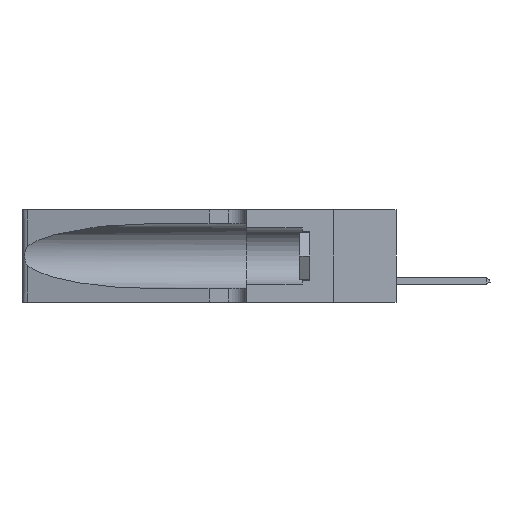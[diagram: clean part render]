
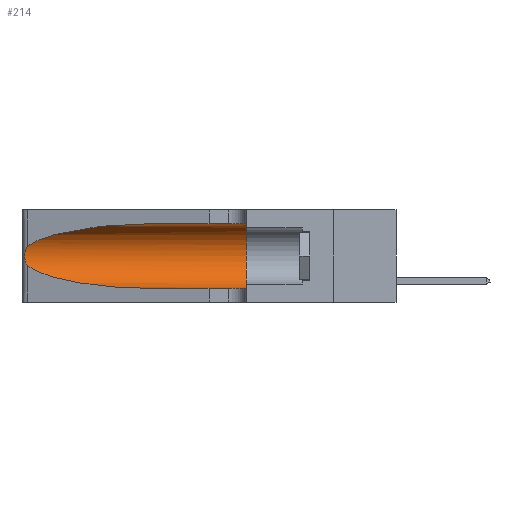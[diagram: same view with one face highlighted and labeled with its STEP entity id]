
A CAD part, left-side view. The second image highlights one B-rep face of the part: STEP entity #214.
In plain terms, the highlighted cylindrical face has radius 3.308 mm (diameter 6.617 mm), a partial arc.
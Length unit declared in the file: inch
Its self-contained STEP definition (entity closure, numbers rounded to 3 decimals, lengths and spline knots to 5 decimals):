
#214 = ADVANCED_FACE ( 'NONE', ( #5492 ), #4150, .F. ) ;
#510 = DIRECTION ( 'NONE',  ( 0., -1., 0. ) ) ;
#840 = CARTESIAN_POINT ( 'NONE',  ( 0.1305, 1.61858, 0.185 ) ) ;
#856 = VECTOR ( 'NONE', #5465, 39.37008 ) ;
#900 = ORIENTED_EDGE ( 'NONE', *, *, #8862, .F. ) ;
#1445 = ORIENTED_EDGE ( 'NONE', *, *, #20544, .T. ) ;
#1498 = AXIS2_PLACEMENT_3D ( 'NONE', #840, #18114, #11240 ) ;
#1716 = ORIENTED_EDGE ( 'NONE', *, *, #21447, .T. ) ;
#1896 = CARTESIAN_POINT ( 'NONE',  ( 0.1305, 1.61858, 0.05475 ) ) ;
#2707 = CARTESIAN_POINT ( 'NONE',  ( 0.25487, 1.22718, 0.14631 ) ) ;
#2871 = ORIENTED_EDGE ( 'NONE', *, *, #12090, .T. ) ;
#3190 = CARTESIAN_POINT ( 'NONE',  ( 0.25639, 1.23184, 0.21858 ) ) ;
#3364 =( BOUNDED_CURVE ( )  B_SPLINE_CURVE ( 3, ( #4228, #4074, #5873, #16490 ),
 .UNSPECIFIED., .F., .F. ) 
 B_SPLINE_CURVE_WITH_KNOTS ( ( 4, 4 ),
 ( 1.5708, 2.84003 ),
 .UNSPECIFIED. ) 
 CURVE ( )  GEOMETRIC_REPRESENTATION_ITEM ( )  RATIONAL_B_SPLINE_CURVE ( ( 1., 0.87, 0.87, 1. ) ) 
 REPRESENTATION_ITEM ( '' )  );
#3707 = CARTESIAN_POINT ( 'NONE',  ( 0.1305, 1.61858, 0.31525 ) ) ;
#4074 = CARTESIAN_POINT ( 'NONE',  ( 0.18966, 0.96281, 0.31525 ) ) ;
#4150 = CYLINDRICAL_SURFACE ( 'NONE', #1498, 0.13025 ) ;
#4228 = CARTESIAN_POINT ( 'NONE',  ( 0.1305, 0.72297, 0.31525 ) ) ;
#5065 = EDGE_CURVE ( 'NONE', #10031, #9863, #18889, .T. ) ;
#5465 = DIRECTION ( 'NONE',  ( 0., -1., 0. ) ) ;
#5492 = FACE_OUTER_BOUND ( 'NONE', #17828, .T. ) ;
#5762 = CARTESIAN_POINT ( 'NONE',  ( 0.1305, 0.35, 0.05475 ) ) ;
#5873 = CARTESIAN_POINT ( 'NONE',  ( 0.2373, 1.15595, 0.28018 ) ) ;
#6160 = CARTESIAN_POINT ( 'NONE',  ( 0.18966, 0.96281, 0.05475 ) ) ;
#6528 = LINE ( 'NONE', #1896, #17446 ) ;
#6623 = CARTESIAN_POINT ( 'NONE',  ( 0.26075, 1.23896, 0.178 ) ) ;
#8283 = CARTESIAN_POINT ( 'NONE',  ( 0.26018, 1.23835, 0.19895 ) ) ;
#8862 = EDGE_CURVE ( 'NONE', #9041, #10031, #13984, .T. ) ;
#9041 = VERTEX_POINT ( 'NONE', #22423 ) ;
#9112 = VERTEX_POINT ( 'NONE', #22352 ) ;
#9363 = VERTEX_POINT ( 'NONE', #14902 ) ;
#9863 = VERTEX_POINT ( 'NONE', #5762 ) ;
#10031 = VERTEX_POINT ( 'NONE', #20386 ) ;
#10655 = CARTESIAN_POINT ( 'NONE',  ( 0.25487, 1.22718, 0.22369 ) ) ;
#11240 = DIRECTION ( 'NONE',  ( 0., 0., -1. ) ) ;
#11399 = CARTESIAN_POINT ( 'NONE',  ( 0.2373, 1.15595, 0.08982 ) ) ;
#11960 = CARTESIAN_POINT ( 'NONE',  ( 0.25854, 1.2359, 0.20912 ) ) ;
#12090 = EDGE_CURVE ( 'NONE', #9041, #21643, #3364, .T. ) ;
#12695 = EDGE_CURVE ( 'NONE', #9363, #9112, #14134, .T. ) ;
#13054 = ORIENTED_EDGE ( 'NONE', *, *, #12695, .T. ) ;
#13269 = AXIS2_PLACEMENT_3D ( 'NONE', #20244, #19953, #22346 ) ;
#13403 = CARTESIAN_POINT ( 'NONE',  ( 0.25639, 1.23186, 0.15144 ) ) ;
#13471 = CARTESIAN_POINT ( 'NONE',  ( 0.25487, 1.22718, 0.14631 ) ) ;
#13553 = ORIENTED_EDGE ( 'NONE', *, *, #5065, .F. ) ;
#13984 = LINE ( 'NONE', #3707, #856 ) ;
#14134 =( BOUNDED_CURVE ( )  B_SPLINE_CURVE ( 3, ( #2707, #11399, #6160, #14930 ),
 .UNSPECIFIED., .F., .F. ) 
 B_SPLINE_CURVE_WITH_KNOTS ( ( 4, 4 ),
 ( 3.44316, 4.71239 ),
 .UNSPECIFIED. ) 
 CURVE ( )  GEOMETRIC_REPRESENTATION_ITEM ( )  RATIONAL_B_SPLINE_CURVE ( ( 1., 0.87, 0.87, 1. ) ) 
 REPRESENTATION_ITEM ( '' )  );
#14902 = CARTESIAN_POINT ( 'NONE',  ( 0.25487, 1.22718, 0.14631 ) ) ;
#14930 = CARTESIAN_POINT ( 'NONE',  ( 0.1305, 0.72297, 0.05475 ) ) ;
#15388 = CARTESIAN_POINT ( 'NONE',  ( 0.26075, 1.23896, 0.19203 ) ) ;
#16490 = CARTESIAN_POINT ( 'NONE',  ( 0.25487, 1.22718, 0.22369 ) ) ;
#16927 = CARTESIAN_POINT ( 'NONE',  ( 0.26017, 1.23833, 0.17102 ) ) ;
#17149 = CARTESIAN_POINT ( 'NONE',  ( 0.25789, 1.23486, 0.15765 ) ) ;
#17446 = VECTOR ( 'NONE', #510, 39.37008 ) ;
#17828 = EDGE_LOOP ( 'NONE', ( #2871, #1716, #13054, #1445, #13553, #900 ) ) ;
#18114 = DIRECTION ( 'NONE',  ( 0., -1., 0. ) ) ;
#18688 = CARTESIAN_POINT ( 'NONE',  ( 0.25856, 1.23593, 0.16098 ) ) ;
#18889 = CIRCLE ( 'NONE', #13269, 0.13025 ) ;
#19580 = B_SPLINE_CURVE_WITH_KNOTS ( 'NONE', 3,
 ( #20342, #22434, #3190, #22360, #11960, #8283, #15388, #6623, #16927, #18688, #17149, #13403, #22210, #13471 ),
 .UNSPECIFIED., .F., .F.,
 ( 4, 2, 2, 2, 2, 2, 4 ),
 ( 0., 0.00027, 0.00053, 0.00107, 0.0016, 0.00187, 0.00214 ),
 .UNSPECIFIED. ) ;
#19953 = DIRECTION ( 'NONE',  ( 0., 1., 0. ) ) ;
#20244 = CARTESIAN_POINT ( 'NONE',  ( 0.1305, 0.35, 0.185 ) ) ;
#20342 = CARTESIAN_POINT ( 'NONE',  ( 0.25487, 1.22718, 0.22369 ) ) ;
#20386 = CARTESIAN_POINT ( 'NONE',  ( 0.1305, 0.35, 0.31525 ) ) ;
#20544 = EDGE_CURVE ( 'NONE', #9112, #9863, #6528, .T. ) ;
#21447 = EDGE_CURVE ( 'NONE', #21643, #9363, #19580, .T. ) ;
#21643 = VERTEX_POINT ( 'NONE', #10655 ) ;
#22210 = CARTESIAN_POINT ( 'NONE',  ( 0.25555, 1.22993, 0.14849 ) ) ;
#22346 = DIRECTION ( 'NONE',  ( 0., 0., 1. ) ) ;
#22352 = CARTESIAN_POINT ( 'NONE',  ( 0.1305, 0.72297, 0.05475 ) ) ;
#22360 = CARTESIAN_POINT ( 'NONE',  ( 0.25787, 1.23484, 0.2124 ) ) ;
#22423 = CARTESIAN_POINT ( 'NONE',  ( 0.1305, 0.72297, 0.31525 ) ) ;
#22434 = CARTESIAN_POINT ( 'NONE',  ( 0.25555, 1.22994, 0.2215 ) ) ;
